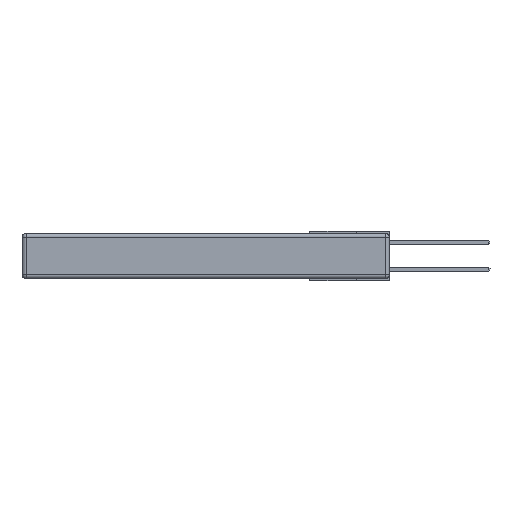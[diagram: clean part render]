
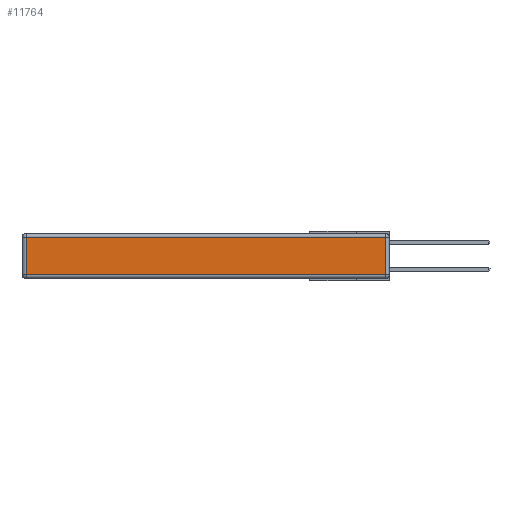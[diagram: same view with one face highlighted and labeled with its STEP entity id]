
A CAD part, left-side view. The second image highlights one B-rep face of the part: STEP entity #11764.
In plain terms, the highlighted planar face has unit normal (-1, 0, 0).
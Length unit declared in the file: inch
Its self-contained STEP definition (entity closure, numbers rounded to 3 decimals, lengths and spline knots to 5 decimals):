
#4071 = AXIS2_PLACEMENT_3D ( 'NONE', #8660, #27084, #13809 ) ;
#4744 = VECTOR ( 'NONE', #32148, 39.37008 ) ;
#6347 = CARTESIAN_POINT ( 'NONE',  ( 0., 2.75, -0.03 ) ) ;
#6636 = EDGE_CURVE ( 'NONE', #8155, #24498, #27295, .T. ) ;
#6771 = DIRECTION ( 'NONE',  ( 0., -1., 0. ) ) ;
#6783 = ORIENTED_EDGE ( 'NONE', *, *, #18175, .T. ) ;
#7823 = VECTOR ( 'NONE', #22118, 39.37008 ) ;
#8155 = VERTEX_POINT ( 'NONE', #20109 ) ;
#8308 = DIRECTION ( 'NONE',  ( 0., 0., -1. ) ) ;
#8660 = CARTESIAN_POINT ( 'NONE',  ( 0., 0., -0.343 ) ) ;
#10594 = VERTEX_POINT ( 'NONE', #14652 ) ;
#11764 = ADVANCED_FACE ( 'NONE', ( #24402 ), #21806, .T. ) ;
#13809 = DIRECTION ( 'NONE',  ( 0., 0., 1. ) ) ;
#14652 = CARTESIAN_POINT ( 'NONE',  ( 0., 2.72, -0.313 ) ) ;
#15100 = LINE ( 'NONE', #26861, #22055 ) ;
#15117 = EDGE_LOOP ( 'NONE', ( #6783, #22620, #26496, #25766 ) ) ;
#16653 = VECTOR ( 'NONE', #6771, 39.37008 ) ;
#17619 = VERTEX_POINT ( 'NONE', #27299 ) ;
#18175 = EDGE_CURVE ( 'NONE', #10594, #8155, #29720, .T. ) ;
#19577 = CARTESIAN_POINT ( 'NONE',  ( 0., 0., -0.313 ) ) ;
#20109 = CARTESIAN_POINT ( 'NONE',  ( 0., 0.03, -0.313 ) ) ;
#21796 = EDGE_CURVE ( 'NONE', #24498, #17619, #33619, .T. ) ;
#21806 = PLANE ( 'NONE',  #4071 ) ;
#22055 = VECTOR ( 'NONE', #8308, 39.37008 ) ;
#22118 = DIRECTION ( 'NONE',  ( 0., 1., 0. ) ) ;
#22620 = ORIENTED_EDGE ( 'NONE', *, *, #6636, .T. ) ;
#24402 = FACE_OUTER_BOUND ( 'NONE', #15117, .T. ) ;
#24498 = VERTEX_POINT ( 'NONE', #30078 ) ;
#25766 = ORIENTED_EDGE ( 'NONE', *, *, #30560, .T. ) ;
#26249 = CARTESIAN_POINT ( 'NONE',  ( 0., 0.03, -0.343 ) ) ;
#26496 = ORIENTED_EDGE ( 'NONE', *, *, #21796, .T. ) ;
#26861 = CARTESIAN_POINT ( 'NONE',  ( 0., 2.72, -0.343 ) ) ;
#27084 = DIRECTION ( 'NONE',  ( -1., 0., 0. ) ) ;
#27295 = LINE ( 'NONE', #26249, #4744 ) ;
#27299 = CARTESIAN_POINT ( 'NONE',  ( 0., 2.72, -0.03 ) ) ;
#29720 = LINE ( 'NONE', #19577, #16653 ) ;
#30078 = CARTESIAN_POINT ( 'NONE',  ( 0., 0.03, -0.03 ) ) ;
#30560 = EDGE_CURVE ( 'NONE', #17619, #10594, #15100, .T. ) ;
#32148 = DIRECTION ( 'NONE',  ( 0., 0., 1. ) ) ;
#33619 = LINE ( 'NONE', #6347, #7823 ) ;
